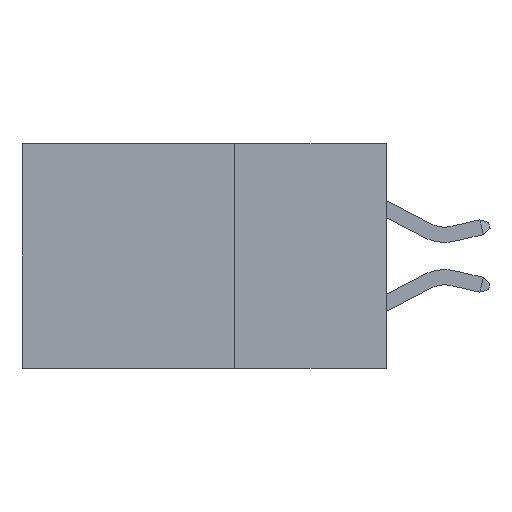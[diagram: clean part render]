
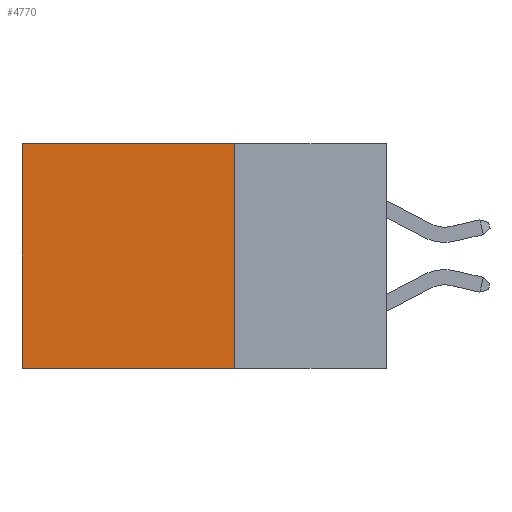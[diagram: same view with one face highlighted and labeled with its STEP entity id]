
A CAD part, left-side view. The second image highlights one B-rep face of the part: STEP entity #4770.
In plain terms, the highlighted planar face has unit normal (-1, 0, 0).
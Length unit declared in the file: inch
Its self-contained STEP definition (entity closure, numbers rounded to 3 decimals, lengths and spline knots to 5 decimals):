
#55 = CARTESIAN_POINT ( 'NONE',  ( 0.298, 0.6, 0. ) ) ;
#445 = DIRECTION ( 'NONE',  ( 0., 1., 0. ) ) ;
#578 = EDGE_CURVE ( 'NONE', #7397, #10850, #3309, .T. ) ;
#826 = VERTEX_POINT ( 'NONE', #55 ) ;
#1618 = LINE ( 'NONE', #6094, #3910 ) ;
#2514 = LINE ( 'NONE', #13097, #10392 ) ;
#2872 = ORIENTED_EDGE ( 'NONE', *, *, #8706, .F. ) ;
#2876 = ORIENTED_EDGE ( 'NONE', *, *, #5439, .T. ) ;
#2950 = FACE_OUTER_BOUND ( 'NONE', #8370, .T. ) ;
#3251 = CARTESIAN_POINT ( 'NONE',  ( 0.298, 0.25, 0. ) ) ;
#3295 = DIRECTION ( 'NONE',  ( 0., 1., 0. ) ) ;
#3309 = LINE ( 'NONE', #7893, #8958 ) ;
#3501 = ORIENTED_EDGE ( 'NONE', *, *, #12492, .T. ) ;
#3910 = VECTOR ( 'NONE', #445, 39.37008 ) ;
#3989 = AXIS2_PLACEMENT_3D ( 'NONE', #9407, #11281, #4718 ) ;
#4302 = LINE ( 'NONE', #3251, #11759 ) ;
#4718 = DIRECTION ( 'NONE',  ( 0., 0., -1. ) ) ;
#4770 = ADVANCED_FACE ( 'NONE', ( #2950 ), #6972, .F. ) ;
#4840 = CARTESIAN_POINT ( 'NONE',  ( 0.298, 0.25, 0. ) ) ;
#4971 = CARTESIAN_POINT ( 'NONE',  ( 0.298, 0.25, -0.37 ) ) ;
#5439 = EDGE_CURVE ( 'NONE', #826, #11488, #2514, .T. ) ;
#6094 = CARTESIAN_POINT ( 'NONE',  ( 0.298, 0.25, -0.37 ) ) ;
#6365 = ORIENTED_EDGE ( 'NONE', *, *, #578, .F. ) ;
#6972 = PLANE ( 'NONE',  #3989 ) ;
#7308 = CARTESIAN_POINT ( 'NONE',  ( 0.298, 0.6, -0.37 ) ) ;
#7397 = VERTEX_POINT ( 'NONE', #4840 ) ;
#7893 = CARTESIAN_POINT ( 'NONE',  ( 0.298, 0.25, 0. ) ) ;
#8035 = DIRECTION ( 'NONE',  ( 0., 0., -1. ) ) ;
#8370 = EDGE_LOOP ( 'NONE', ( #2876, #2872, #6365, #3501 ) ) ;
#8706 = EDGE_CURVE ( 'NONE', #10850, #11488, #1618, .T. ) ;
#8958 = VECTOR ( 'NONE', #8035, 39.37008 ) ;
#9407 = CARTESIAN_POINT ( 'NONE',  ( 0.298, 0.25, 0. ) ) ;
#9951 = DIRECTION ( 'NONE',  ( 0., 0., -1. ) ) ;
#10392 = VECTOR ( 'NONE', #9951, 39.37008 ) ;
#10850 = VERTEX_POINT ( 'NONE', #4971 ) ;
#11281 = DIRECTION ( 'NONE',  ( 1., 0., 0. ) ) ;
#11488 = VERTEX_POINT ( 'NONE', #7308 ) ;
#11759 = VECTOR ( 'NONE', #3295, 39.37008 ) ;
#12492 = EDGE_CURVE ( 'NONE', #7397, #826, #4302, .T. ) ;
#13097 = CARTESIAN_POINT ( 'NONE',  ( 0.298, 0.6, 0. ) ) ;
